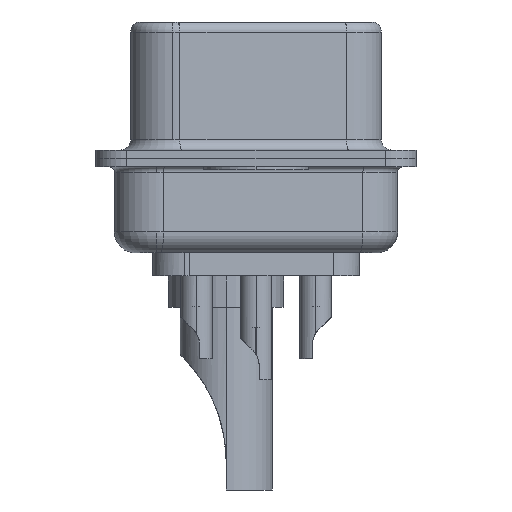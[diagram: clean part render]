
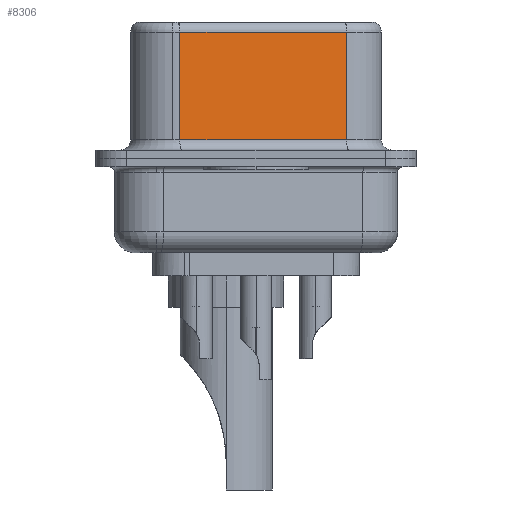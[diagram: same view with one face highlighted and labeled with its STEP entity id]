
A CAD part, left-side view. The second image highlights one B-rep face of the part: STEP entity #8306.
In plain terms, the highlighted planar face has unit normal (-0.985, -0.174, 0).
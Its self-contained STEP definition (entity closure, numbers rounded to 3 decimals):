
#1704 = CARTESIAN_POINT ( 'NONE',  ( 5.132, -4.322, 6.02 ) ) ;
#2080 = EDGE_LOOP ( 'NONE', ( #10403, #12817, #10962, #20586 ) ) ;
#2313 = LINE ( 'NONE', #15975, #12727 ) ;
#2565 = VECTOR ( 'NONE', #8267, 1000. ) ;
#3873 = FACE_OUTER_BOUND ( 'NONE', #2080, .T. ) ;
#4220 = EDGE_CURVE ( 'NONE', #12214, #25298, #13610, .T. ) ;
#4862 = DIRECTION ( 'NONE',  ( 0.174, -0.985, 0. ) ) ;
#5006 = EDGE_CURVE ( 'NONE', #14343, #14870, #7100, .T. ) ;
#6295 = LINE ( 'NONE', #15837, #22237 ) ;
#7100 = LINE ( 'NONE', #25312, #12608 ) ;
#7310 = DIRECTION ( 'NONE',  ( -0.174, 0.985, 0. ) ) ;
#7345 = DIRECTION ( 'NONE',  ( 0.985, 0.174, 0. ) ) ;
#7800 = PLANE ( 'NONE',  #23302 ) ;
#8267 = DIRECTION ( 'NONE',  ( -0.174, 0.985, 0. ) ) ;
#8306 = ADVANCED_FACE ( 'NONE', ( #3873 ), #7800, .F. ) ;
#8455 = CARTESIAN_POINT ( 'NONE',  ( 5.132, -4.322, 6.52 ) ) ;
#10403 = ORIENTED_EDGE ( 'NONE', *, *, #18708, .F. ) ;
#10962 = ORIENTED_EDGE ( 'NONE', *, *, #17483, .T. ) ;
#12214 = VERTEX_POINT ( 'NONE', #20209 ) ;
#12608 = VECTOR ( 'NONE', #4862, 1000. ) ;
#12727 = VECTOR ( 'NONE', #16158, 1000. ) ;
#12817 = ORIENTED_EDGE ( 'NONE', *, *, #4220, .T. ) ;
#13610 = LINE ( 'NONE', #1704, #2565 ) ;
#14343 = VERTEX_POINT ( 'NONE', #26685 ) ;
#14870 = VERTEX_POINT ( 'NONE', #20047 ) ;
#15837 = CARTESIAN_POINT ( 'NONE',  ( 3.73, 3.628, 6.52 ) ) ;
#15975 = CARTESIAN_POINT ( 'NONE',  ( 5.132, -4.322, 6.52 ) ) ;
#16158 = DIRECTION ( 'NONE',  ( 0., 0., -1. ) ) ;
#17483 = EDGE_CURVE ( 'NONE', #25298, #14343, #6295, .T. ) ;
#18708 = EDGE_CURVE ( 'NONE', #12214, #14870, #2313, .T. ) ;
#20033 = DIRECTION ( 'NONE',  ( 0., 0., -1. ) ) ;
#20047 = CARTESIAN_POINT ( 'NONE',  ( 5.132, -4.322, 0.9 ) ) ;
#20209 = CARTESIAN_POINT ( 'NONE',  ( 5.132, -4.322, 6.02 ) ) ;
#20586 = ORIENTED_EDGE ( 'NONE', *, *, #5006, .T. ) ;
#22237 = VECTOR ( 'NONE', #20033, 1000. ) ;
#23302 = AXIS2_PLACEMENT_3D ( 'NONE', #8455, #7345, #7310 ) ;
#25298 = VERTEX_POINT ( 'NONE', #25823 ) ;
#25312 = CARTESIAN_POINT ( 'NONE',  ( 5.132, -4.322, 0.9 ) ) ;
#25823 = CARTESIAN_POINT ( 'NONE',  ( 3.73, 3.628, 6.02 ) ) ;
#26685 = CARTESIAN_POINT ( 'NONE',  ( 3.73, 3.628, 0.9 ) ) ;
